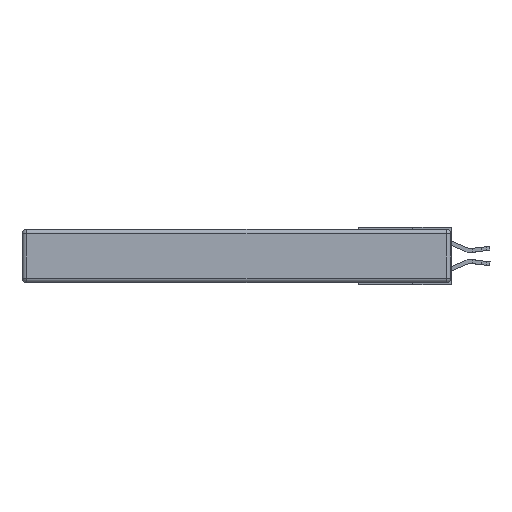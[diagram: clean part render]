
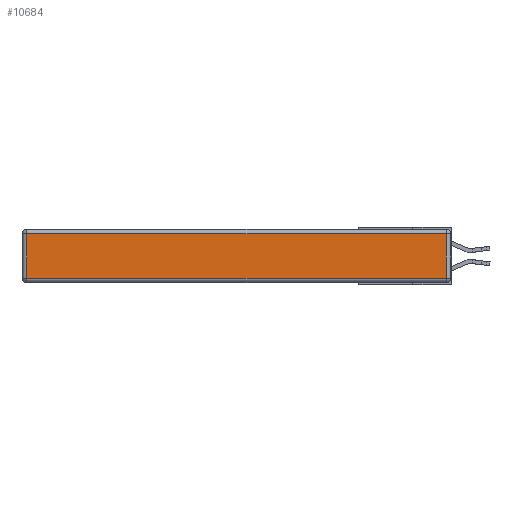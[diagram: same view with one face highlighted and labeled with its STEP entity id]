
A CAD part, left-side view. The second image highlights one B-rep face of the part: STEP entity #10684.
In plain terms, the highlighted planar face has unit normal (-1, 0, 0).
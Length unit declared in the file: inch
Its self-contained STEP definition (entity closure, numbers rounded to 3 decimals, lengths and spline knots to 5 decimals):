
#1609 = VERTEX_POINT ( 'NONE', #16079 ) ;
#1964 = AXIS2_PLACEMENT_3D ( 'NONE', #17065, #12902, #19185 ) ;
#2227 = ORIENTED_EDGE ( 'NONE', *, *, #21700, .T. ) ;
#3429 = CARTESIAN_POINT ( 'NONE',  ( 0., 2.75, -0.03 ) ) ;
#4919 = LINE ( 'NONE', #3429, #19723 ) ;
#5119 = CARTESIAN_POINT ( 'NONE',  ( 0., 2.72, -0.343 ) ) ;
#5251 = VERTEX_POINT ( 'NONE', #8489 ) ;
#5583 = VECTOR ( 'NONE', #26314, 39.37008 ) ;
#5663 = FACE_OUTER_BOUND ( 'NONE', #17685, .T. ) ;
#6651 = PLANE ( 'NONE',  #1964 ) ;
#6663 = ORIENTED_EDGE ( 'NONE', *, *, #6981, .T. ) ;
#6981 = EDGE_CURVE ( 'NONE', #18350, #7987, #15850, .T. ) ;
#7987 = VERTEX_POINT ( 'NONE', #19644 ) ;
#8489 = CARTESIAN_POINT ( 'NONE',  ( 0., 2.72, -0.03 ) ) ;
#10668 = VECTOR ( 'NONE', #13142, 39.37008 ) ;
#10684 = ADVANCED_FACE ( 'NONE', ( #5663 ), #6651, .T. ) ;
#11034 = CARTESIAN_POINT ( 'NONE',  ( 0., 0.03, -0.343 ) ) ;
#12874 = VECTOR ( 'NONE', #25807, 39.37008 ) ;
#12902 = DIRECTION ( 'NONE',  ( -1., 0., 0. ) ) ;
#13142 = DIRECTION ( 'NONE',  ( 0., -1., 0. ) ) ;
#15454 = CARTESIAN_POINT ( 'NONE',  ( 0., 0., -0.313 ) ) ;
#15850 = LINE ( 'NONE', #11034, #12874 ) ;
#16079 = CARTESIAN_POINT ( 'NONE',  ( 0., 2.72, -0.313 ) ) ;
#16282 = LINE ( 'NONE', #15454, #10668 ) ;
#17065 = CARTESIAN_POINT ( 'NONE',  ( 0., 0., -0.343 ) ) ;
#17552 = ORIENTED_EDGE ( 'NONE', *, *, #25998, .T. ) ;
#17663 = EDGE_CURVE ( 'NONE', #1609, #18350, #16282, .T. ) ;
#17685 = EDGE_LOOP ( 'NONE', ( #25470, #6663, #2227, #17552 ) ) ;
#18156 = DIRECTION ( 'NONE',  ( 0., 1., 0. ) ) ;
#18350 = VERTEX_POINT ( 'NONE', #20651 ) ;
#19078 = LINE ( 'NONE', #5119, #5583 ) ;
#19185 = DIRECTION ( 'NONE',  ( 0., 0., 1. ) ) ;
#19644 = CARTESIAN_POINT ( 'NONE',  ( 0., 0.03, -0.03 ) ) ;
#19723 = VECTOR ( 'NONE', #18156, 39.37008 ) ;
#20651 = CARTESIAN_POINT ( 'NONE',  ( 0., 0.03, -0.313 ) ) ;
#21700 = EDGE_CURVE ( 'NONE', #7987, #5251, #4919, .T. ) ;
#25470 = ORIENTED_EDGE ( 'NONE', *, *, #17663, .T. ) ;
#25807 = DIRECTION ( 'NONE',  ( 0., 0., 1. ) ) ;
#25998 = EDGE_CURVE ( 'NONE', #5251, #1609, #19078, .T. ) ;
#26314 = DIRECTION ( 'NONE',  ( 0., 0., -1. ) ) ;
